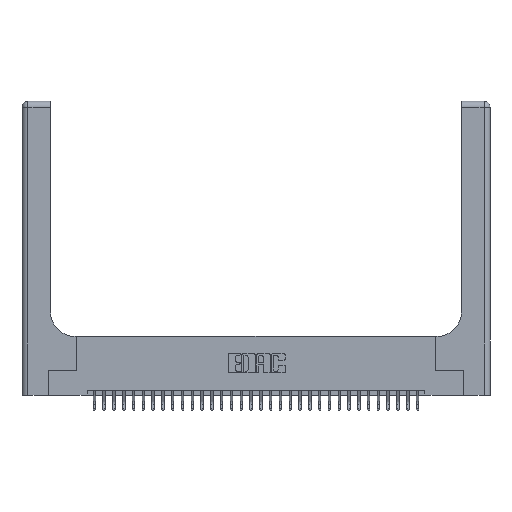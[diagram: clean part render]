
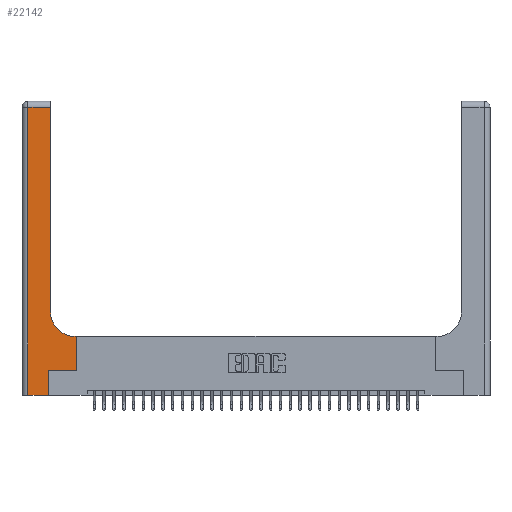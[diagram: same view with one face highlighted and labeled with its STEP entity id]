
A CAD part, top view. The second image highlights one B-rep face of the part: STEP entity #22142.
In plain terms, the highlighted planar face has unit normal (0, 0, 1).
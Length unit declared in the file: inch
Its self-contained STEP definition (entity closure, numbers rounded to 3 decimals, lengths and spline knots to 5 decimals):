
#534 = CARTESIAN_POINT ( 'NONE',  ( 0.269, 0.25, 0.37 ) ) ;
#1196 = VECTOR ( 'NONE', #21670, 39.37008 ) ;
#1389 = LINE ( 'NONE', #27715, #14215 ) ;
#1852 = VECTOR ( 'NONE', #10771, 39.37008 ) ;
#1922 = VERTEX_POINT ( 'NONE', #20393 ) ;
#3015 = VERTEX_POINT ( 'NONE', #6700 ) ;
#3157 = CARTESIAN_POINT ( 'NONE',  ( 0.5585, 0.6, 0.37 ) ) ;
#3506 = LINE ( 'NONE', #3511, #10310 ) ;
#3511 = CARTESIAN_POINT ( 'NONE',  ( 0.06, 3., 0.37 ) ) ;
#3694 = ORIENTED_EDGE ( 'NONE', *, *, #12436, .T. ) ;
#4527 = FACE_OUTER_BOUND ( 'NONE', #30282, .T. ) ;
#4736 = PLANE ( 'NONE',  #5407 ) ;
#5383 = CARTESIAN_POINT ( 'NONE',  ( 0.5585, 0.25, 0.37 ) ) ;
#5407 = AXIS2_PLACEMENT_3D ( 'NONE', #20132, #22711, #7414 ) ;
#5414 = CARTESIAN_POINT ( 'NONE',  ( 0.5415, 0.85, 0.37 ) ) ;
#5753 = VECTOR ( 'NONE', #15132, 39.37008 ) ;
#5910 = VERTEX_POINT ( 'NONE', #7849 ) ;
#6120 = CARTESIAN_POINT ( 'NONE',  ( 0., 0., 0.37 ) ) ;
#6183 = EDGE_CURVE ( 'NONE', #6874, #23730, #14826, .T. ) ;
#6700 = CARTESIAN_POINT ( 'NONE',  ( 0.06, 2.94, 0.37 ) ) ;
#6874 = VERTEX_POINT ( 'NONE', #3157 ) ;
#7136 = EDGE_CURVE ( 'NONE', #8927, #31873, #1389, .T. ) ;
#7414 = DIRECTION ( 'NONE',  ( -1., 0., 0. ) ) ;
#7849 = CARTESIAN_POINT ( 'NONE',  ( 0.2915, 2.94, 0.37 ) ) ;
#7968 = DIRECTION ( 'NONE',  ( 1., 0., 0. ) ) ;
#8504 = VECTOR ( 'NONE', #21679, 39.37008 ) ;
#8687 = DIRECTION ( 'NONE',  ( 1., 0., 0. ) ) ;
#8927 = VERTEX_POINT ( 'NONE', #21847 ) ;
#10125 = LINE ( 'NONE', #29297, #8504 ) ;
#10310 = VECTOR ( 'NONE', #31572, 39.37008 ) ;
#10771 = DIRECTION ( 'NONE',  ( -1., 0., 0. ) ) ;
#11333 = ORIENTED_EDGE ( 'NONE', *, *, #27050, .T. ) ;
#11635 = AXIS2_PLACEMENT_3D ( 'NONE', #5414, #23278, #7968 ) ;
#12436 = EDGE_CURVE ( 'NONE', #3015, #1922, #3506, .T. ) ;
#12570 = CARTESIAN_POINT ( 'NONE',  ( 0.2915, 3., 0.37 ) ) ;
#13328 = ORIENTED_EDGE ( 'NONE', *, *, #7136, .T. ) ;
#13351 = CARTESIAN_POINT ( 'NONE',  ( 0., 2.94, 0.37 ) ) ;
#14185 = VECTOR ( 'NONE', #15868, 39.37008 ) ;
#14215 = VECTOR ( 'NONE', #30284, 39.37008 ) ;
#14400 = CIRCLE ( 'NONE', #11635, 0.25 ) ;
#14826 = LINE ( 'NONE', #19108, #1196 ) ;
#15006 = EDGE_CURVE ( 'NONE', #1922, #8927, #32262, .T. ) ;
#15132 = DIRECTION ( 'NONE',  ( 0., 1., 0. ) ) ;
#15789 = LINE ( 'NONE', #534, #14185 ) ;
#15868 = DIRECTION ( 'NONE',  ( 1., 0., 0. ) ) ;
#16312 = EDGE_CURVE ( 'NONE', #31873, #18697, #15789, .T. ) ;
#17544 = CARTESIAN_POINT ( 'NONE',  ( 0.2915, 0.85, 0.37 ) ) ;
#17693 = ORIENTED_EDGE ( 'NONE', *, *, #16312, .T. ) ;
#18638 = VECTOR ( 'NONE', #8687, 39.37008 ) ;
#18697 = VERTEX_POINT ( 'NONE', #5383 ) ;
#19053 = ORIENTED_EDGE ( 'NONE', *, *, #22438, .T. ) ;
#19108 = CARTESIAN_POINT ( 'NONE',  ( 0.2915, 0.6, 0.37 ) ) ;
#19249 = ORIENTED_EDGE ( 'NONE', *, *, #15006, .T. ) ;
#20132 = CARTESIAN_POINT ( 'NONE',  ( 0., 3., 0.37 ) ) ;
#20393 = CARTESIAN_POINT ( 'NONE',  ( 0.06, 0., 0.37 ) ) ;
#21670 = DIRECTION ( 'NONE',  ( -1., 0., 0. ) ) ;
#21679 = DIRECTION ( 'NONE',  ( 0., 1., 0. ) ) ;
#21847 = CARTESIAN_POINT ( 'NONE',  ( 0.269, 0., 0.37 ) ) ;
#22142 = ADVANCED_FACE ( 'NONE', ( #4527 ), #4736, .F. ) ;
#22438 = EDGE_CURVE ( 'NONE', #18697, #6874, #10125, .T. ) ;
#22711 = DIRECTION ( 'NONE',  ( 0., 0., -1. ) ) ;
#23278 = DIRECTION ( 'NONE',  ( 0., 0., -1. ) ) ;
#23730 = VERTEX_POINT ( 'NONE', #24063 ) ;
#24063 = CARTESIAN_POINT ( 'NONE',  ( 0.5415, 0.6, 0.37 ) ) ;
#25176 = ORIENTED_EDGE ( 'NONE', *, *, #26043, .T. ) ;
#26043 = EDGE_CURVE ( 'NONE', #5910, #3015, #29863, .T. ) ;
#26122 = LINE ( 'NONE', #12570, #5753 ) ;
#26324 = ORIENTED_EDGE ( 'NONE', *, *, #6183, .T. ) ;
#27050 = EDGE_CURVE ( 'NONE', #23730, #27514, #14400, .T. ) ;
#27514 = VERTEX_POINT ( 'NONE', #17544 ) ;
#27715 = CARTESIAN_POINT ( 'NONE',  ( 0.269, 0., 0.37 ) ) ;
#29297 = CARTESIAN_POINT ( 'NONE',  ( 0.5585, 0.25, 0.37 ) ) ;
#29863 = LINE ( 'NONE', #13351, #1852 ) ;
#30282 = EDGE_LOOP ( 'NONE', ( #32301, #25176, #3694, #19249, #13328, #17693, #19053, #26324, #11333 ) ) ;
#30284 = DIRECTION ( 'NONE',  ( 0., 1., 0. ) ) ;
#30557 = EDGE_CURVE ( 'NONE', #27514, #5910, #26122, .T. ) ;
#31572 = DIRECTION ( 'NONE',  ( 0., -1., 0. ) ) ;
#31873 = VERTEX_POINT ( 'NONE', #32720 ) ;
#32262 = LINE ( 'NONE', #6120, #18638 ) ;
#32301 = ORIENTED_EDGE ( 'NONE', *, *, #30557, .T. ) ;
#32720 = CARTESIAN_POINT ( 'NONE',  ( 0.269, 0.25, 0.37 ) ) ;
